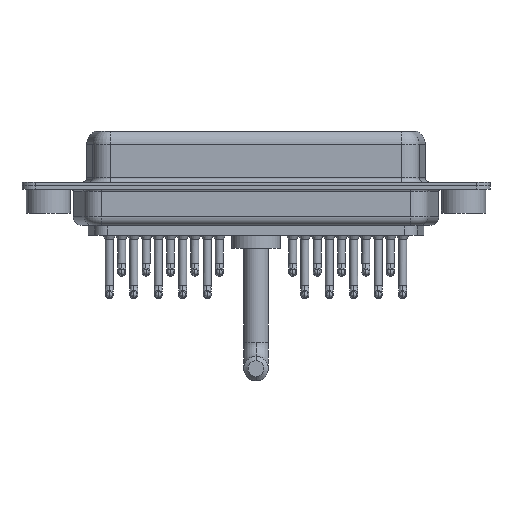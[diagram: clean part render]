
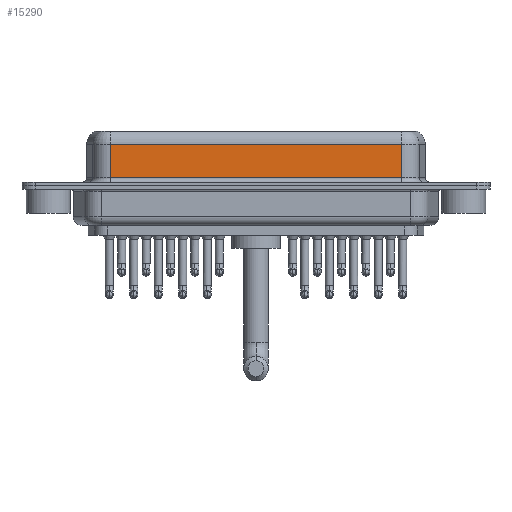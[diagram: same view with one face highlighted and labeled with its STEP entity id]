
A CAD part, front view. The second image highlights one B-rep face of the part: STEP entity #15290.
In plain terms, the highlighted planar face has unit normal (0, -1, 0).
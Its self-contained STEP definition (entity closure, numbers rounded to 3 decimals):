
#627 = PLANE ( 'NONE',  #19180 ) ;
#1811 = ORIENTED_EDGE ( 'NONE', *, *, #22190, .F. ) ;
#2225 = CARTESIAN_POINT ( 'NONE',  ( 40.037, -3.95, 6.4 ) ) ;
#2678 = ORIENTED_EDGE ( 'NONE', *, *, #13959, .T. ) ;
#3266 = VERTEX_POINT ( 'NONE', #6771 ) ;
#3975 = VECTOR ( 'NONE', #16795, 1000. ) ;
#6523 = DIRECTION ( 'NONE',  ( -1., 0., 0. ) ) ;
#6771 = CARTESIAN_POINT ( 'NONE',  ( 7.013, -3.95, 0.9 ) ) ;
#7314 = CARTESIAN_POINT ( 'NONE',  ( 7.013, -3.95, 4.65 ) ) ;
#7479 = DIRECTION ( 'NONE',  ( 0., 1., 0. ) ) ;
#7572 = ORIENTED_EDGE ( 'NONE', *, *, #14668, .T. ) ;
#7641 = LINE ( 'NONE', #14738, #3975 ) ;
#8071 = VECTOR ( 'NONE', #21733, 1000. ) ;
#10075 = LINE ( 'NONE', #15555, #12597 ) ;
#10202 = VERTEX_POINT ( 'NONE', #19124 ) ;
#10739 = CARTESIAN_POINT ( 'NONE',  ( 40.037, -3.95, 0.9 ) ) ;
#10920 = DIRECTION ( 'NONE',  ( 0., 0., 1. ) ) ;
#10978 = EDGE_CURVE ( 'NONE', #3266, #20095, #7641, .T. ) ;
#11137 = DIRECTION ( 'NONE',  ( 0., 0., -1. ) ) ;
#12521 = VECTOR ( 'NONE', #11137, 1000. ) ;
#12597 = VECTOR ( 'NONE', #6523, 1000. ) ;
#13737 = CARTESIAN_POINT ( 'NONE',  ( 40.037, -3.95, 6.4 ) ) ;
#13959 = EDGE_CURVE ( 'NONE', #14914, #3266, #14240, .T. ) ;
#14240 = LINE ( 'NONE', #14458, #12521 ) ;
#14458 = CARTESIAN_POINT ( 'NONE',  ( 7.013, -3.95, 6.4 ) ) ;
#14668 = EDGE_CURVE ( 'NONE', #10202, #14914, #10075, .T. ) ;
#14738 = CARTESIAN_POINT ( 'NONE',  ( 40.037, -3.95, 0.9 ) ) ;
#14914 = VERTEX_POINT ( 'NONE', #7314 ) ;
#15290 = ADVANCED_FACE ( 'NONE', ( #19498 ), #627, .F. ) ;
#15555 = CARTESIAN_POINT ( 'NONE',  ( 40.037, -3.95, 4.65 ) ) ;
#15912 = LINE ( 'NONE', #13737, #8071 ) ;
#16042 = ORIENTED_EDGE ( 'NONE', *, *, #10978, .T. ) ;
#16795 = DIRECTION ( 'NONE',  ( 1., 0., 0. ) ) ;
#16895 = EDGE_LOOP ( 'NONE', ( #1811, #7572, #2678, #16042 ) ) ;
#19124 = CARTESIAN_POINT ( 'NONE',  ( 40.037, -3.95, 4.65 ) ) ;
#19180 = AXIS2_PLACEMENT_3D ( 'NONE', #2225, #7479, #10920 ) ;
#19498 = FACE_OUTER_BOUND ( 'NONE', #16895, .T. ) ;
#20095 = VERTEX_POINT ( 'NONE', #10739 ) ;
#21733 = DIRECTION ( 'NONE',  ( 0., 0., -1. ) ) ;
#22190 = EDGE_CURVE ( 'NONE', #10202, #20095, #15912, .T. ) ;
